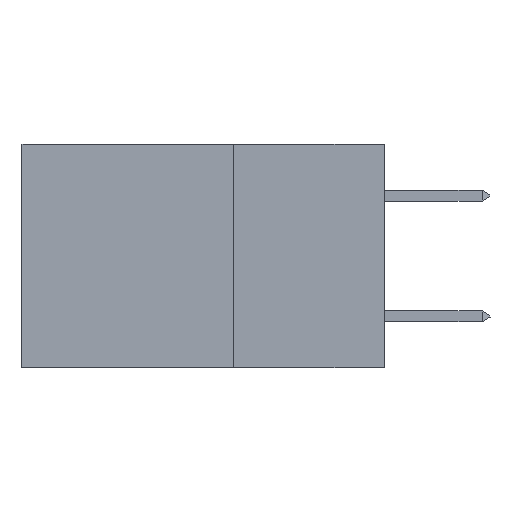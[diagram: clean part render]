
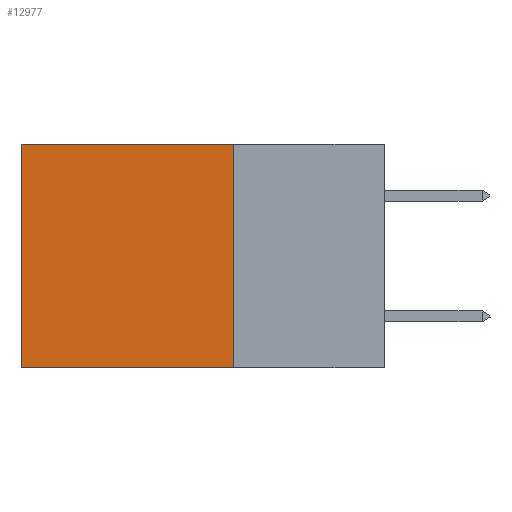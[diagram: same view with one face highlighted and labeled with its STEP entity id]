
A CAD part, left-side view. The second image highlights one B-rep face of the part: STEP entity #12977.
In plain terms, the highlighted planar face has unit normal (-1, 0, 0).
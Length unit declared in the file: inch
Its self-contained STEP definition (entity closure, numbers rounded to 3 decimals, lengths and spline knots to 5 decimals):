
#2843 = EDGE_CURVE ( 'NONE', #30023, #21981, #27645, .T. ) ;
#4419 = ORIENTED_EDGE ( 'NONE', *, *, #13542, .F. ) ;
#4559 = CARTESIAN_POINT ( 'NONE',  ( 0.2875, 0.6, 0. ) ) ;
#5051 = EDGE_LOOP ( 'NONE', ( #29955, #4419, #29034, #31955 ) ) ;
#6667 = CARTESIAN_POINT ( 'NONE',  ( 0.2875, 0.25, 0. ) ) ;
#7651 = VECTOR ( 'NONE', #11346, 39.37008 ) ;
#8165 = AXIS2_PLACEMENT_3D ( 'NONE', #6667, #9376, #27803 ) ;
#8562 = EDGE_CURVE ( 'NONE', #18476, #33038, #9468, .T. ) ;
#8595 = CARTESIAN_POINT ( 'NONE',  ( 0.2875, 0.6, 0. ) ) ;
#9376 = DIRECTION ( 'NONE',  ( 1., 0., 0. ) ) ;
#9468 = LINE ( 'NONE', #4559, #15829 ) ;
#10231 = FACE_OUTER_BOUND ( 'NONE', #5051, .T. ) ;
#11346 = DIRECTION ( 'NONE',  ( 0., 1., 0. ) ) ;
#12977 = ADVANCED_FACE ( 'NONE', ( #10231 ), #22616, .F. ) ;
#13542 = EDGE_CURVE ( 'NONE', #21981, #33038, #14839, .T. ) ;
#13969 = CARTESIAN_POINT ( 'NONE',  ( 0.2875, 0.25, -0.37 ) ) ;
#14839 = LINE ( 'NONE', #13969, #7651 ) ;
#14997 = LINE ( 'NONE', #17193, #15851 ) ;
#15472 = DIRECTION ( 'NONE',  ( 0., 0., -1. ) ) ;
#15829 = VECTOR ( 'NONE', #15472, 39.37008 ) ;
#15851 = VECTOR ( 'NONE', #32711, 39.37008 ) ;
#17193 = CARTESIAN_POINT ( 'NONE',  ( 0.2875, 0.25, 0. ) ) ;
#18476 = VERTEX_POINT ( 'NONE', #8595 ) ;
#18623 = CARTESIAN_POINT ( 'NONE',  ( 0.2875, 0.25, -0.37 ) ) ;
#20444 = EDGE_CURVE ( 'NONE', #30023, #18476, #14997, .T. ) ;
#20783 = VECTOR ( 'NONE', #31612, 39.37008 ) ;
#21981 = VERTEX_POINT ( 'NONE', #18623 ) ;
#22616 = PLANE ( 'NONE',  #8165 ) ;
#23726 = CARTESIAN_POINT ( 'NONE',  ( 0.2875, 0.6, -0.37 ) ) ;
#27645 = LINE ( 'NONE', #32278, #20783 ) ;
#27803 = DIRECTION ( 'NONE',  ( 0., 0., -1. ) ) ;
#29034 = ORIENTED_EDGE ( 'NONE', *, *, #2843, .F. ) ;
#29955 = ORIENTED_EDGE ( 'NONE', *, *, #8562, .T. ) ;
#30023 = VERTEX_POINT ( 'NONE', #32892 ) ;
#31612 = DIRECTION ( 'NONE',  ( 0., 0., -1. ) ) ;
#31955 = ORIENTED_EDGE ( 'NONE', *, *, #20444, .T. ) ;
#32278 = CARTESIAN_POINT ( 'NONE',  ( 0.2875, 0.25, 0. ) ) ;
#32711 = DIRECTION ( 'NONE',  ( 0., 1., 0. ) ) ;
#32892 = CARTESIAN_POINT ( 'NONE',  ( 0.2875, 0.25, 0. ) ) ;
#33038 = VERTEX_POINT ( 'NONE', #23726 ) ;
